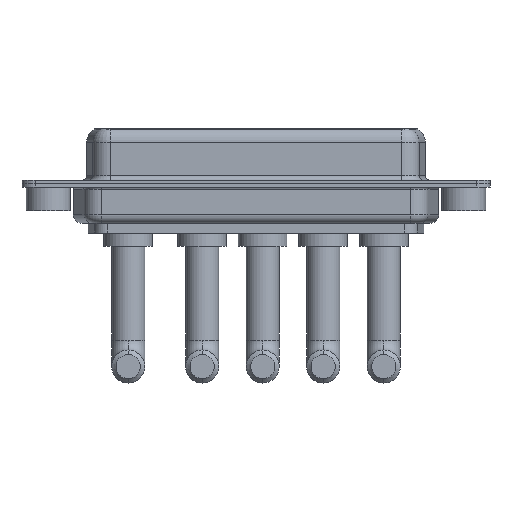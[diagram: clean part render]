
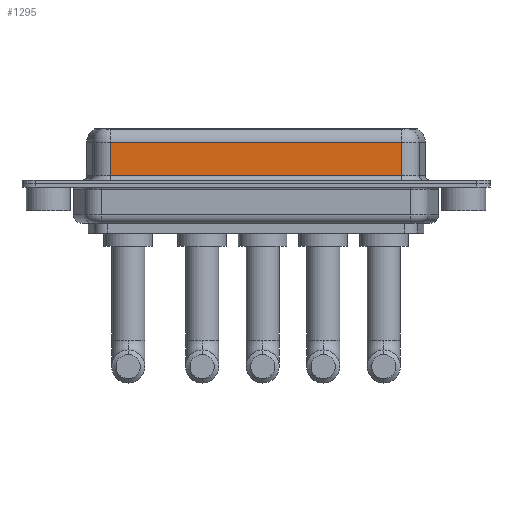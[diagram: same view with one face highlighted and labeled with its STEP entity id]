
A CAD part, front view. The second image highlights one B-rep face of the part: STEP entity #1295.
In plain terms, the highlighted planar face has unit normal (0, -1, 0).
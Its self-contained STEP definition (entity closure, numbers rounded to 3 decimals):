
#55 = DIRECTION ( 'NONE',  ( 0., 0., -1. ) ) ;
#939 = VECTOR ( 'NONE', #10890, 1000. ) ;
#1083 = ORIENTED_EDGE ( 'NONE', *, *, #5579, .T. ) ;
#1169 = LINE ( 'NONE', #2062, #11218 ) ;
#1193 = ORIENTED_EDGE ( 'NONE', *, *, #11679, .T. ) ;
#1295 = ADVANCED_FACE ( 'NONE', ( #1853 ), #12641, .F. ) ;
#1562 = VERTEX_POINT ( 'NONE', #3701 ) ;
#1853 = FACE_OUTER_BOUND ( 'NONE', #11234, .T. ) ;
#2062 = CARTESIAN_POINT ( 'NONE',  ( 40.037, -3.95, 4.65 ) ) ;
#2315 = CARTESIAN_POINT ( 'NONE',  ( 40.037, -3.95, 4.65 ) ) ;
#3303 = AXIS2_PLACEMENT_3D ( 'NONE', #7556, #10761, #12451 ) ;
#3430 = VERTEX_POINT ( 'NONE', #10641 ) ;
#3701 = CARTESIAN_POINT ( 'NONE',  ( 7.013, -3.95, 0.9 ) ) ;
#3749 = DIRECTION ( 'NONE',  ( 1., 0., 0. ) ) ;
#4842 = VERTEX_POINT ( 'NONE', #2315 ) ;
#4853 = CARTESIAN_POINT ( 'NONE',  ( 7.013, -3.95, 6.4 ) ) ;
#5579 = EDGE_CURVE ( 'NONE', #7587, #1562, #11862, .T. ) ;
#5626 = EDGE_CURVE ( 'NONE', #4842, #3430, #7817, .T. ) ;
#5817 = CARTESIAN_POINT ( 'NONE',  ( 40.037, -3.95, 6.4 ) ) ;
#6664 = VECTOR ( 'NONE', #55, 1000. ) ;
#6964 = ORIENTED_EDGE ( 'NONE', *, *, #9230, .T. ) ;
#7122 = DIRECTION ( 'NONE',  ( -1., 0., 0. ) ) ;
#7358 = CARTESIAN_POINT ( 'NONE',  ( 7.013, -3.95, 4.65 ) ) ;
#7556 = CARTESIAN_POINT ( 'NONE',  ( 40.037, -3.95, 6.4 ) ) ;
#7587 = VERTEX_POINT ( 'NONE', #7358 ) ;
#7817 = LINE ( 'NONE', #5817, #939 ) ;
#9230 = EDGE_CURVE ( 'NONE', #4842, #7587, #1169, .T. ) ;
#10533 = CARTESIAN_POINT ( 'NONE',  ( 40.037, -3.95, 0.9 ) ) ;
#10633 = VECTOR ( 'NONE', #3749, 1000. ) ;
#10641 = CARTESIAN_POINT ( 'NONE',  ( 40.037, -3.95, 0.9 ) ) ;
#10761 = DIRECTION ( 'NONE',  ( 0., 1., 0. ) ) ;
#10890 = DIRECTION ( 'NONE',  ( 0., 0., -1. ) ) ;
#11077 = ORIENTED_EDGE ( 'NONE', *, *, #5626, .F. ) ;
#11218 = VECTOR ( 'NONE', #7122, 1000. ) ;
#11234 = EDGE_LOOP ( 'NONE', ( #11077, #6964, #1083, #1193 ) ) ;
#11522 = LINE ( 'NONE', #10533, #10633 ) ;
#11679 = EDGE_CURVE ( 'NONE', #1562, #3430, #11522, .T. ) ;
#11862 = LINE ( 'NONE', #4853, #6664 ) ;
#12451 = DIRECTION ( 'NONE',  ( 0., 0., 1. ) ) ;
#12641 = PLANE ( 'NONE',  #3303 ) ;
